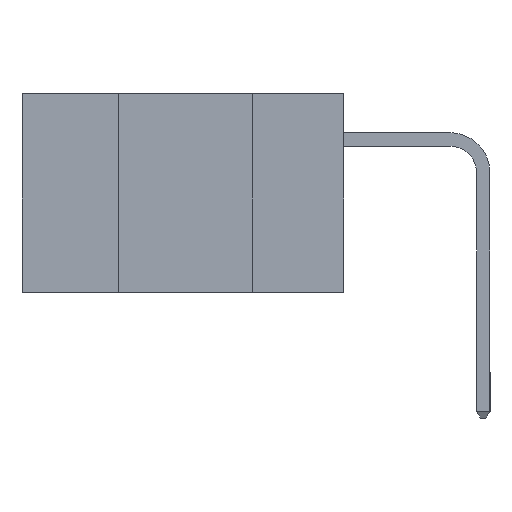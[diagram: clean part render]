
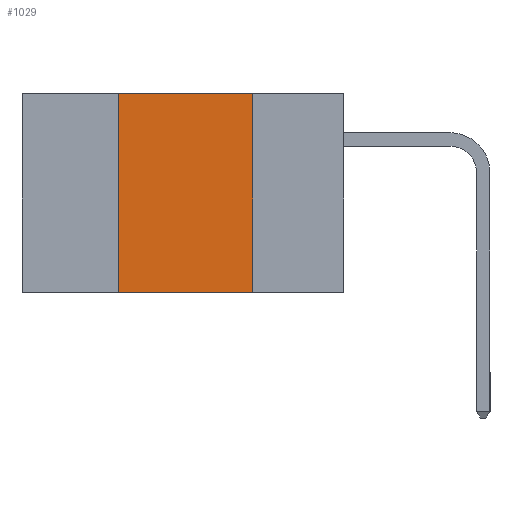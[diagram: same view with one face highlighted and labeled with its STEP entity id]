
A CAD part, left-side view. The second image highlights one B-rep face of the part: STEP entity #1029.
In plain terms, the highlighted planar face has unit normal (-1, 0, 0).
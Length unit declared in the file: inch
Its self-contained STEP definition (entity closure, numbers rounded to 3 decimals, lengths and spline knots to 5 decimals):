
#231 = DIRECTION ( 'NONE',  ( 0., 0., -1. ) ) ;
#340 = DIRECTION ( 'NONE',  ( 0., 0., -1. ) ) ;
#1029 = ADVANCED_FACE ( 'NONE', ( #20057 ), #17433, .F. ) ;
#1184 = LINE ( 'NONE', #2381, #4433 ) ;
#2361 = CARTESIAN_POINT ( 'NONE',  ( 0., 0.42, -0.37 ) ) ;
#2381 = CARTESIAN_POINT ( 'NONE',  ( 0., 0.17, 0. ) ) ;
#2433 = VECTOR ( 'NONE', #4541, 39.37008 ) ;
#2447 = EDGE_CURVE ( 'NONE', #11611, #9593, #1184, .T. ) ;
#2690 = ORIENTED_EDGE ( 'NONE', *, *, #2447, .F. ) ;
#2793 = CARTESIAN_POINT ( 'NONE',  ( 0., 0.6, 0. ) ) ;
#3115 = LINE ( 'NONE', #6356, #5479 ) ;
#3605 = CARTESIAN_POINT ( 'NONE',  ( 0., 0.17, -0.37 ) ) ;
#3613 = ORIENTED_EDGE ( 'NONE', *, *, #21703, .T. ) ;
#3758 = ORIENTED_EDGE ( 'NONE', *, *, #17546, .F. ) ;
#4058 = VERTEX_POINT ( 'NONE', #5426 ) ;
#4433 = VECTOR ( 'NONE', #231, 39.37008 ) ;
#4523 = LINE ( 'NONE', #2793, #2433 ) ;
#4541 = DIRECTION ( 'NONE',  ( 0., -1., 0. ) ) ;
#5426 = CARTESIAN_POINT ( 'NONE',  ( 0., 0.42, 0. ) ) ;
#5461 = CARTESIAN_POINT ( 'NONE',  ( 0., 0.6, -0.37 ) ) ;
#5479 = VECTOR ( 'NONE', #17720, 39.37008 ) ;
#5844 = ORIENTED_EDGE ( 'NONE', *, *, #22248, .F. ) ;
#6356 = CARTESIAN_POINT ( 'NONE',  ( 0., 0.42, 0. ) ) ;
#8740 = VECTOR ( 'NONE', #20739, 39.37008 ) ;
#9421 = CARTESIAN_POINT ( 'NONE',  ( 0., 0.17, 0. ) ) ;
#9593 = VERTEX_POINT ( 'NONE', #3605 ) ;
#9654 = EDGE_LOOP ( 'NONE', ( #2690, #5844, #3758, #3613 ) ) ;
#11611 = VERTEX_POINT ( 'NONE', #9421 ) ;
#13375 = AXIS2_PLACEMENT_3D ( 'NONE', #19349, #23329, #340 ) ;
#17433 = PLANE ( 'NONE',  #13375 ) ;
#17546 = EDGE_CURVE ( 'NONE', #23151, #4058, #3115, .T. ) ;
#17720 = DIRECTION ( 'NONE',  ( 0., 0., 1. ) ) ;
#18897 = LINE ( 'NONE', #5461, #8740 ) ;
#19349 = CARTESIAN_POINT ( 'NONE',  ( 0., 0.6, 0. ) ) ;
#20057 = FACE_OUTER_BOUND ( 'NONE', #9654, .T. ) ;
#20739 = DIRECTION ( 'NONE',  ( 0., -1., 0. ) ) ;
#21703 = EDGE_CURVE ( 'NONE', #23151, #9593, #18897, .T. ) ;
#22248 = EDGE_CURVE ( 'NONE', #4058, #11611, #4523, .T. ) ;
#23151 = VERTEX_POINT ( 'NONE', #2361 ) ;
#23329 = DIRECTION ( 'NONE',  ( 1., 0., 0. ) ) ;
